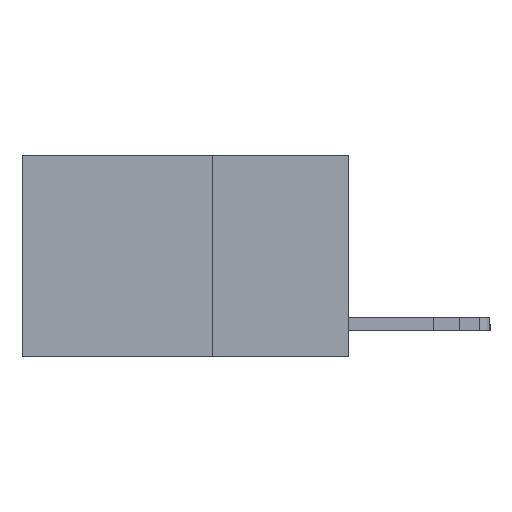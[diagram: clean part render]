
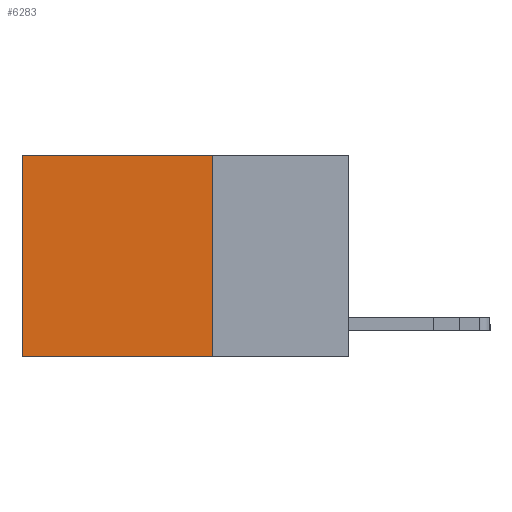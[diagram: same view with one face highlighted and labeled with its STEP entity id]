
A CAD part, left-side view. The second image highlights one B-rep face of the part: STEP entity #6283.
In plain terms, the highlighted planar face has unit normal (-1, 0, 0).
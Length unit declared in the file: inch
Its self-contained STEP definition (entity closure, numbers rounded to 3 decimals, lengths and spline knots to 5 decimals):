
#245 = CARTESIAN_POINT ( 'NONE',  ( 0.2625, 0.25, 0. ) ) ;
#247 = LINE ( 'NONE', #15252, #11335 ) ;
#358 = DIRECTION ( 'NONE',  ( 0., 1., 0. ) ) ;
#379 = ORIENTED_EDGE ( 'NONE', *, *, #9418, .F. ) ;
#721 = VERTEX_POINT ( 'NONE', #3433 ) ;
#1291 = VECTOR ( 'NONE', #11645, 39.37008 ) ;
#3013 = DIRECTION ( 'NONE',  ( 0., 0., -1. ) ) ;
#3433 = CARTESIAN_POINT ( 'NONE',  ( 0.2625, 0.25, -0.37 ) ) ;
#5496 = ORIENTED_EDGE ( 'NONE', *, *, #8129, .T. ) ;
#5592 = LINE ( 'NONE', #13112, #10934 ) ;
#5619 = AXIS2_PLACEMENT_3D ( 'NONE', #14051, #15022, #3013 ) ;
#5656 = VERTEX_POINT ( 'NONE', #9197 ) ;
#6253 = ORIENTED_EDGE ( 'NONE', *, *, #7784, .T. ) ;
#6283 = ADVANCED_FACE ( 'NONE', ( #15359 ), #6717, .F. ) ;
#6717 = PLANE ( 'NONE',  #5619 ) ;
#6753 = EDGE_CURVE ( 'NONE', #15822, #721, #247, .T. ) ;
#7705 = VERTEX_POINT ( 'NONE', #13035 ) ;
#7784 = EDGE_CURVE ( 'NONE', #15822, #5656, #5592, .T. ) ;
#8129 = EDGE_CURVE ( 'NONE', #5656, #7705, #12672, .T. ) ;
#9197 = CARTESIAN_POINT ( 'NONE',  ( 0.2625, 0.6, 0. ) ) ;
#9418 = EDGE_CURVE ( 'NONE', #721, #7705, #11513, .T. ) ;
#10934 = VECTOR ( 'NONE', #12954, 39.37008 ) ;
#11335 = VECTOR ( 'NONE', #11562, 39.37008 ) ;
#11428 = CARTESIAN_POINT ( 'NONE',  ( 0.2625, 0.25, -0.37 ) ) ;
#11513 = LINE ( 'NONE', #11428, #12757 ) ;
#11562 = DIRECTION ( 'NONE',  ( 0., 0., -1. ) ) ;
#11645 = DIRECTION ( 'NONE',  ( 0., 0., -1. ) ) ;
#12504 = EDGE_LOOP ( 'NONE', ( #5496, #379, #15321, #6253 ) ) ;
#12672 = LINE ( 'NONE', #12756, #1291 ) ;
#12756 = CARTESIAN_POINT ( 'NONE',  ( 0.2625, 0.6, 0. ) ) ;
#12757 = VECTOR ( 'NONE', #358, 39.37008 ) ;
#12954 = DIRECTION ( 'NONE',  ( 0., 1., 0. ) ) ;
#13035 = CARTESIAN_POINT ( 'NONE',  ( 0.2625, 0.6, -0.37 ) ) ;
#13112 = CARTESIAN_POINT ( 'NONE',  ( 0.2625, 0.25, 0. ) ) ;
#14051 = CARTESIAN_POINT ( 'NONE',  ( 0.2625, 0.25, 0. ) ) ;
#15022 = DIRECTION ( 'NONE',  ( 1., 0., 0. ) ) ;
#15252 = CARTESIAN_POINT ( 'NONE',  ( 0.2625, 0.25, 0. ) ) ;
#15321 = ORIENTED_EDGE ( 'NONE', *, *, #6753, .F. ) ;
#15359 = FACE_OUTER_BOUND ( 'NONE', #12504, .T. ) ;
#15822 = VERTEX_POINT ( 'NONE', #245 ) ;
